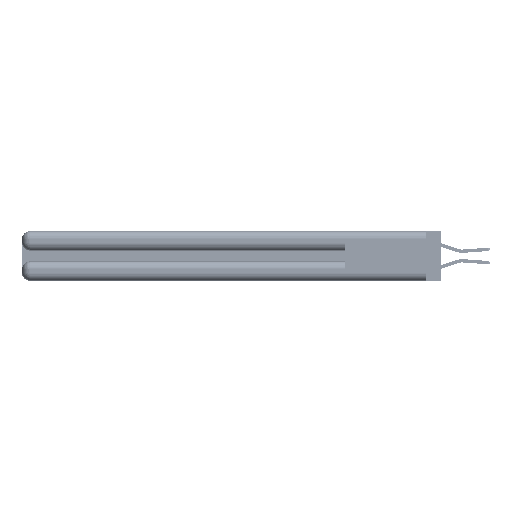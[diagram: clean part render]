
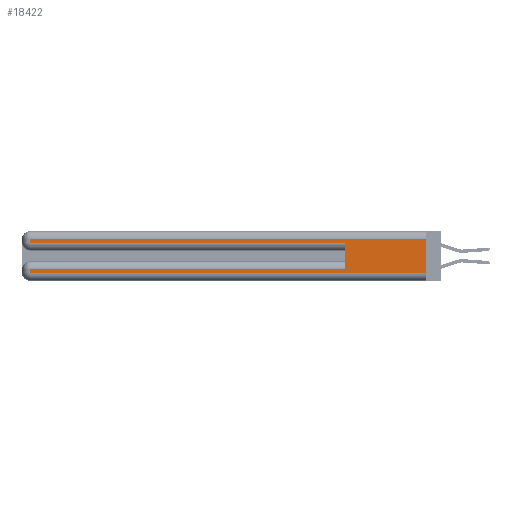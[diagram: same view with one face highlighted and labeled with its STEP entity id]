
A CAD part, left-side view. The second image highlights one B-rep face of the part: STEP entity #18422.
In plain terms, the highlighted planar face has unit normal (-1, 0, 0).
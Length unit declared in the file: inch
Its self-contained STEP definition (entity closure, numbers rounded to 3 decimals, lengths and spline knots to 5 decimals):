
#650 = VECTOR ( 'NONE', #35531, 39.37008 ) ;
#2709 = CARTESIAN_POINT ( 'NONE',  ( 0., 0., 0.085 ) ) ;
#3332 = FACE_OUTER_BOUND ( 'NONE', #55827, .T. ) ;
#4095 = LINE ( 'NONE', #23937, #45974 ) ;
#4953 = ORIENTED_EDGE ( 'NONE', *, *, #54456, .F. ) ;
#5216 = CARTESIAN_POINT ( 'NONE',  ( 0., 0., 0.06 ) ) ;
#7747 = ORIENTED_EDGE ( 'NONE', *, *, #9911, .T. ) ;
#7792 = VERTEX_POINT ( 'NONE', #35709 ) ;
#8255 = CARTESIAN_POINT ( 'NONE',  ( 0., 0., 0.31 ) ) ;
#9048 = VERTEX_POINT ( 'NONE', #27260 ) ;
#9103 = LINE ( 'NONE', #21404, #42243 ) ;
#9628 = CARTESIAN_POINT ( 'NONE',  ( 0., 0.6, 0.145 ) ) ;
#9736 = CARTESIAN_POINT ( 'NONE',  ( 0., 2.94, 0.31 ) ) ;
#9911 = EDGE_CURVE ( 'NONE', #30124, #26339, #4095, .T. ) ;
#10794 = VECTOR ( 'NONE', #47169, 39.37008 ) ;
#11132 = DIRECTION ( 'NONE',  ( 0., -1., 0. ) ) ;
#17178 = VECTOR ( 'NONE', #18611, 39.37008 ) ;
#17272 = DIRECTION ( 'NONE',  ( 1., 0., 0. ) ) ;
#18422 = ADVANCED_FACE ( 'NONE', ( #3332 ), #19515, .F. ) ;
#18429 = LINE ( 'NONE', #55622, #19772 ) ;
#18527 = LINE ( 'NONE', #35862, #17178 ) ;
#18611 = DIRECTION ( 'NONE',  ( 0., 0., -1. ) ) ;
#19071 = CARTESIAN_POINT ( 'NONE',  ( 0., 0., 0.285 ) ) ;
#19515 = PLANE ( 'NONE',  #36208 ) ;
#19772 = VECTOR ( 'NONE', #25370, 39.37008 ) ;
#21404 = CARTESIAN_POINT ( 'NONE',  ( 0., 0., 0.37 ) ) ;
#21557 = ORIENTED_EDGE ( 'NONE', *, *, #31185, .T. ) ;
#23856 = ORIENTED_EDGE ( 'NONE', *, *, #46003, .T. ) ;
#23937 = CARTESIAN_POINT ( 'NONE',  ( 0., 0., 0.06 ) ) ;
#25370 = DIRECTION ( 'NONE',  ( 0., 0., -1. ) ) ;
#26339 = VERTEX_POINT ( 'NONE', #5216 ) ;
#27260 = CARTESIAN_POINT ( 'NONE',  ( 0., 2.94, 0.285 ) ) ;
#29482 = LINE ( 'NONE', #2709, #39614 ) ;
#30124 = VERTEX_POINT ( 'NONE', #30812 ) ;
#30642 = CARTESIAN_POINT ( 'NONE',  ( 0., 0., 0.31 ) ) ;
#30812 = CARTESIAN_POINT ( 'NONE',  ( 0., 2.94, 0.06 ) ) ;
#31185 = EDGE_CURVE ( 'NONE', #47934, #52275, #45284, .T. ) ;
#31962 = DIRECTION ( 'NONE',  ( 0., -1., 0. ) ) ;
#32906 = DIRECTION ( 'NONE',  ( 0., 1., 0. ) ) ;
#34443 = EDGE_CURVE ( 'NONE', #9048, #7792, #53697, .T. ) ;
#34477 = ORIENTED_EDGE ( 'NONE', *, *, #37896, .T. ) ;
#34882 = CARTESIAN_POINT ( 'NONE',  ( 0., 0.6, 0.085 ) ) ;
#35531 = DIRECTION ( 'NONE',  ( 0., 0., 1. ) ) ;
#35709 = CARTESIAN_POINT ( 'NONE',  ( 0., 0.6, 0.285 ) ) ;
#35862 = CARTESIAN_POINT ( 'NONE',  ( 0., 2.94, 0.37 ) ) ;
#36208 = AXIS2_PLACEMENT_3D ( 'NONE', #43196, #17272, #47535 ) ;
#37896 = EDGE_CURVE ( 'NONE', #52275, #9048, #18527, .T. ) ;
#39614 = VECTOR ( 'NONE', #32906, 39.37008 ) ;
#40858 = VECTOR ( 'NONE', #31962, 39.37008 ) ;
#42243 = VECTOR ( 'NONE', #47337, 39.37008 ) ;
#42629 = ORIENTED_EDGE ( 'NONE', *, *, #34443, .T. ) ;
#43196 = CARTESIAN_POINT ( 'NONE',  ( 0., 0., 0.37 ) ) ;
#44438 = EDGE_CURVE ( 'NONE', #50187, #53044, #29482, .T. ) ;
#45244 = LINE ( 'NONE', #9628, #650 ) ;
#45284 = LINE ( 'NONE', #8255, #10794 ) ;
#45974 = VECTOR ( 'NONE', #11132, 39.37008 ) ;
#45997 = ORIENTED_EDGE ( 'NONE', *, *, #49131, .F. ) ;
#46003 = EDGE_CURVE ( 'NONE', #53044, #30124, #18429, .T. ) ;
#47169 = DIRECTION ( 'NONE',  ( 0., 1., 0. ) ) ;
#47337 = DIRECTION ( 'NONE',  ( 0., 0., -1. ) ) ;
#47535 = DIRECTION ( 'NONE',  ( 0., 0., -1. ) ) ;
#47934 = VERTEX_POINT ( 'NONE', #30642 ) ;
#49131 = EDGE_CURVE ( 'NONE', #47934, #26339, #9103, .T. ) ;
#49876 = ORIENTED_EDGE ( 'NONE', *, *, #44438, .T. ) ;
#50187 = VERTEX_POINT ( 'NONE', #34882 ) ;
#51338 = CARTESIAN_POINT ( 'NONE',  ( 0., 2.94, 0.085 ) ) ;
#52275 = VERTEX_POINT ( 'NONE', #9736 ) ;
#53044 = VERTEX_POINT ( 'NONE', #51338 ) ;
#53697 = LINE ( 'NONE', #19071, #40858 ) ;
#54456 = EDGE_CURVE ( 'NONE', #50187, #7792, #45244, .T. ) ;
#55622 = CARTESIAN_POINT ( 'NONE',  ( 0., 2.94, 0.37 ) ) ;
#55827 = EDGE_LOOP ( 'NONE', ( #45997, #21557, #34477, #42629, #4953, #49876, #23856, #7747 ) ) ;
